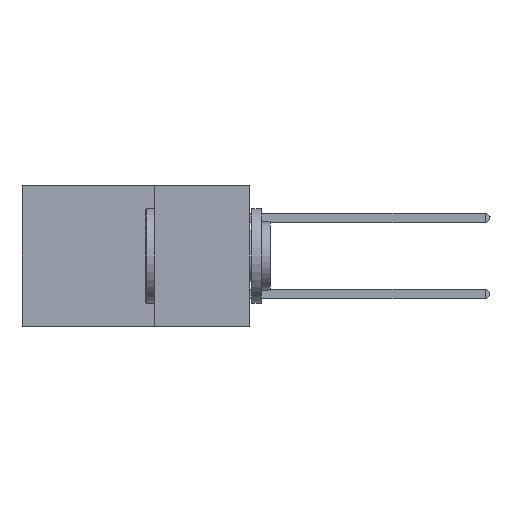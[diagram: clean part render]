
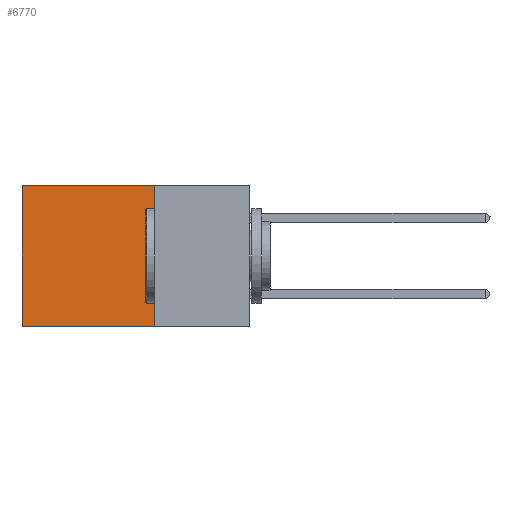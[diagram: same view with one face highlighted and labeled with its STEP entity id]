
A CAD part, left-side view. The second image highlights one B-rep face of the part: STEP entity #6770.
In plain terms, the highlighted planar face has unit normal (-1, 0, 0).
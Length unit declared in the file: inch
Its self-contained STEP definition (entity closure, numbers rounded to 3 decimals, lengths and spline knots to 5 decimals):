
#191 = LINE ( 'NONE', #6486, #6655 ) ;
#342 = CARTESIAN_POINT ( 'NONE',  ( 0.2875, 0.6, 0. ) ) ;
#435 = DIRECTION ( 'NONE',  ( 0., 0., -1. ) ) ;
#503 = VERTEX_POINT ( 'NONE', #4910 ) ;
#755 = CARTESIAN_POINT ( 'NONE',  ( 0.2875, 0.25, -0.37 ) ) ;
#1300 = ORIENTED_EDGE ( 'NONE', *, *, #6882, .F. ) ;
#1692 = ORIENTED_EDGE ( 'NONE', *, *, #7131, .T. ) ;
#3184 = EDGE_CURVE ( 'NONE', #5830, #503, #6478, .T. ) ;
#3837 = VERTEX_POINT ( 'NONE', #10803 ) ;
#3938 = VERTEX_POINT ( 'NONE', #10109 ) ;
#4910 = CARTESIAN_POINT ( 'NONE',  ( 0.2875, 0.6, -0.37 ) ) ;
#5830 = VERTEX_POINT ( 'NONE', #755 ) ;
#6110 = VECTOR ( 'NONE', #15435, 39.37008 ) ;
#6478 = LINE ( 'NONE', #15404, #6110 ) ;
#6486 = CARTESIAN_POINT ( 'NONE',  ( 0.2875, 0.25, 0. ) ) ;
#6522 = DIRECTION ( 'NONE',  ( 0., 1., 0. ) ) ;
#6655 = VECTOR ( 'NONE', #6522, 39.37008 ) ;
#6770 = ADVANCED_FACE ( 'NONE', ( #8699 ), #10463, .F. ) ;
#6882 = EDGE_CURVE ( 'NONE', #3837, #5830, #11401, .T. ) ;
#7131 = EDGE_CURVE ( 'NONE', #3837, #3938, #191, .T. ) ;
#7229 = VECTOR ( 'NONE', #9336, 39.37008 ) ;
#7701 = EDGE_CURVE ( 'NONE', #3938, #503, #12062, .T. ) ;
#8699 = FACE_OUTER_BOUND ( 'NONE', #13985, .T. ) ;
#9230 = CARTESIAN_POINT ( 'NONE',  ( 0.2875, 0.25, 0. ) ) ;
#9336 = DIRECTION ( 'NONE',  ( 0., 0., -1. ) ) ;
#10109 = CARTESIAN_POINT ( 'NONE',  ( 0.2875, 0.6, 0. ) ) ;
#10384 = DIRECTION ( 'NONE',  ( 0., 0., -1. ) ) ;
#10387 = DIRECTION ( 'NONE',  ( 1., 0., 0. ) ) ;
#10443 = CARTESIAN_POINT ( 'NONE',  ( 0.2875, 0.25, 0. ) ) ;
#10452 = ORIENTED_EDGE ( 'NONE', *, *, #3184, .F. ) ;
#10463 = PLANE ( 'NONE',  #11840 ) ;
#10803 = CARTESIAN_POINT ( 'NONE',  ( 0.2875, 0.25, 0. ) ) ;
#11401 = LINE ( 'NONE', #9230, #7229 ) ;
#11614 = ORIENTED_EDGE ( 'NONE', *, *, #7701, .T. ) ;
#11840 = AXIS2_PLACEMENT_3D ( 'NONE', #10443, #10387, #10384 ) ;
#12062 = LINE ( 'NONE', #342, #14597 ) ;
#13985 = EDGE_LOOP ( 'NONE', ( #11614, #10452, #1300, #1692 ) ) ;
#14597 = VECTOR ( 'NONE', #435, 39.37008 ) ;
#15404 = CARTESIAN_POINT ( 'NONE',  ( 0.2875, 0.25, -0.37 ) ) ;
#15435 = DIRECTION ( 'NONE',  ( 0., 1., 0. ) ) ;
